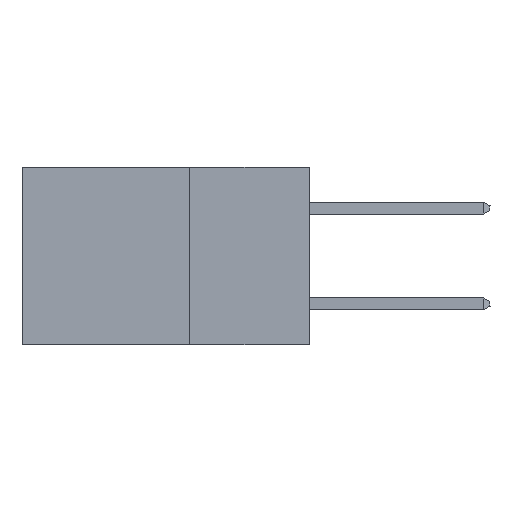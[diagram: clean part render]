
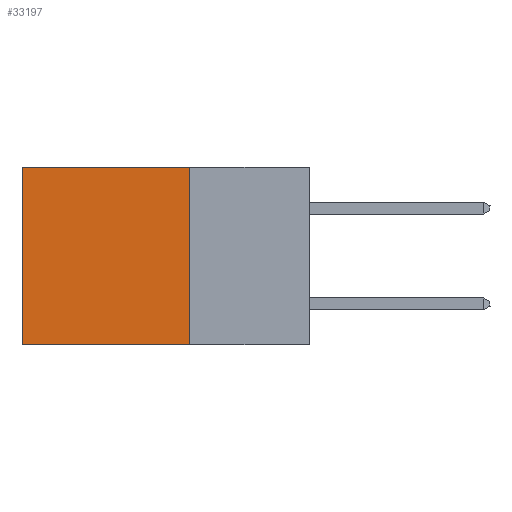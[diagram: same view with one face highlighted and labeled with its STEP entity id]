
A CAD part, left-side view. The second image highlights one B-rep face of the part: STEP entity #33197.
In plain terms, the highlighted planar face has unit normal (-1, 0, 0).
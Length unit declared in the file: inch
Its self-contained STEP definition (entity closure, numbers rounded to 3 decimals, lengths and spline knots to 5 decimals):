
#730 = CARTESIAN_POINT ( 'NONE',  ( 0.2875, 0.25, 0. ) ) ;
#1878 = ORIENTED_EDGE ( 'NONE', *, *, #35398, .F. ) ;
#3039 = EDGE_LOOP ( 'NONE', ( #25379, #34932, #1878, #5384 ) ) ;
#4183 = VERTEX_POINT ( 'NONE', #28457 ) ;
#4563 = VECTOR ( 'NONE', #16544, 39.37008 ) ;
#5384 = ORIENTED_EDGE ( 'NONE', *, *, #29564, .T. ) ;
#5754 = DIRECTION ( 'NONE',  ( 1., 0., 0. ) ) ;
#7189 = FACE_OUTER_BOUND ( 'NONE', #3039, .T. ) ;
#7534 = VERTEX_POINT ( 'NONE', #20396 ) ;
#7854 = LINE ( 'NONE', #38084, #27688 ) ;
#12444 = EDGE_CURVE ( 'NONE', #4183, #32822, #7854, .T. ) ;
#12642 = DIRECTION ( 'NONE',  ( 0., 1., 0. ) ) ;
#15235 = LINE ( 'NONE', #25444, #4563 ) ;
#15278 = VECTOR ( 'NONE', #12642, 39.37008 ) ;
#16068 = DIRECTION ( 'NONE',  ( 0., 1., 0. ) ) ;
#16188 = DIRECTION ( 'NONE',  ( 0., 0., -1. ) ) ;
#16544 = DIRECTION ( 'NONE',  ( 0., 0., -1. ) ) ;
#18367 = CARTESIAN_POINT ( 'NONE',  ( 0.2875, 0.25, 0. ) ) ;
#20396 = CARTESIAN_POINT ( 'NONE',  ( 0.2875, 0.25, -0.37 ) ) ;
#21008 = VECTOR ( 'NONE', #16068, 39.37008 ) ;
#21527 = LINE ( 'NONE', #31007, #15278 ) ;
#22448 = CARTESIAN_POINT ( 'NONE',  ( 0.2875, 0.6, -0.37 ) ) ;
#23914 = PLANE ( 'NONE',  #38702 ) ;
#25379 = ORIENTED_EDGE ( 'NONE', *, *, #12444, .T. ) ;
#25444 = CARTESIAN_POINT ( 'NONE',  ( 0.2875, 0.25, 0. ) ) ;
#26979 = CARTESIAN_POINT ( 'NONE',  ( 0.2875, 0.25, 0. ) ) ;
#27688 = VECTOR ( 'NONE', #16188, 39.37008 ) ;
#27789 = DIRECTION ( 'NONE',  ( 0., 0., -1. ) ) ;
#28457 = CARTESIAN_POINT ( 'NONE',  ( 0.2875, 0.6, 0. ) ) ;
#29564 = EDGE_CURVE ( 'NONE', #37608, #4183, #34116, .T. ) ;
#31007 = CARTESIAN_POINT ( 'NONE',  ( 0.2875, 0.25, -0.37 ) ) ;
#32822 = VERTEX_POINT ( 'NONE', #22448 ) ;
#33197 = ADVANCED_FACE ( 'NONE', ( #7189 ), #23914, .F. ) ;
#34116 = LINE ( 'NONE', #730, #21008 ) ;
#34932 = ORIENTED_EDGE ( 'NONE', *, *, #35095, .F. ) ;
#35095 = EDGE_CURVE ( 'NONE', #7534, #32822, #21527, .T. ) ;
#35398 = EDGE_CURVE ( 'NONE', #37608, #7534, #15235, .T. ) ;
#37608 = VERTEX_POINT ( 'NONE', #18367 ) ;
#38084 = CARTESIAN_POINT ( 'NONE',  ( 0.2875, 0.6, 0. ) ) ;
#38702 = AXIS2_PLACEMENT_3D ( 'NONE', #26979, #5754, #27789 ) ;
